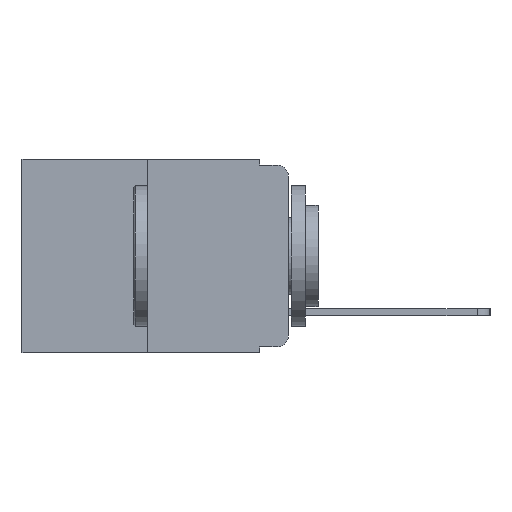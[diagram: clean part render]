
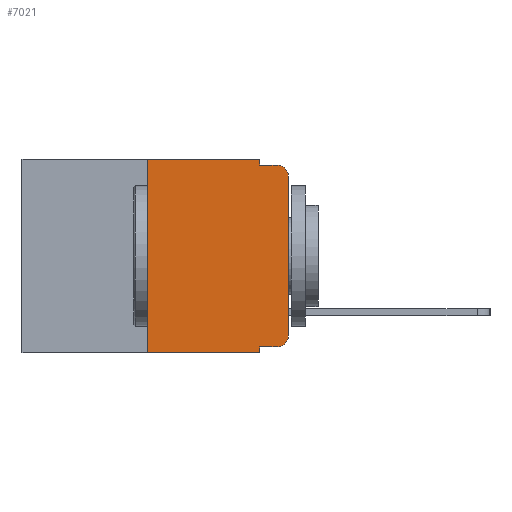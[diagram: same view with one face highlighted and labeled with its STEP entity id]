
A CAD part, left-side view. The second image highlights one B-rep face of the part: STEP entity #7021.
In plain terms, the highlighted planar face has unit normal (-1, 0, 0).
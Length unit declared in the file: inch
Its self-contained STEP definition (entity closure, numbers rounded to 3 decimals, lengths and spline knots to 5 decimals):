
#21 = CARTESIAN_POINT ( 'NONE',  ( 0., 0.473, 0. ) ) ;
#171 = LINE ( 'NONE', #21, #10136 ) ;
#456 = LINE ( 'NONE', #12877, #19580 ) ;
#613 = EDGE_CURVE ( 'NONE', #20553, #6563, #11273, .T. ) ;
#792 = VECTOR ( 'NONE', #21512, 39.37008 ) ;
#1247 = DIRECTION ( 'NONE',  ( 0., 0., -1. ) ) ;
#1403 = VERTEX_POINT ( 'NONE', #15650 ) ;
#1652 = VERTEX_POINT ( 'NONE', #16987 ) ;
#2051 = CARTESIAN_POINT ( 'NONE',  ( 0., 0.02, -0.01 ) ) ;
#2196 = VERTEX_POINT ( 'NONE', #22762 ) ;
#2244 = LINE ( 'NONE', #10944, #20990 ) ;
#2334 = ORIENTED_EDGE ( 'NONE', *, *, #5971, .T. ) ;
#3184 = CARTESIAN_POINT ( 'NONE',  ( 0., 0.473, 0. ) ) ;
#3349 = EDGE_CURVE ( 'NONE', #6563, #7145, #6574, .T. ) ;
#3550 = ORIENTED_EDGE ( 'NONE', *, *, #4656, .T. ) ;
#3631 = ORIENTED_EDGE ( 'NONE', *, *, #3349, .F. ) ;
#4011 = CARTESIAN_POINT ( 'NONE',  ( 0., 0.051, 0. ) ) ;
#4197 = ORIENTED_EDGE ( 'NONE', *, *, #613, .F. ) ;
#4545 = ORIENTED_EDGE ( 'NONE', *, *, #21954, .F. ) ;
#4577 = VERTEX_POINT ( 'NONE', #6796 ) ;
#4656 = EDGE_CURVE ( 'NONE', #1403, #7145, #19176, .T. ) ;
#4668 = CIRCLE ( 'NONE', #15121, 0.02 ) ;
#4827 = ORIENTED_EDGE ( 'NONE', *, *, #23019, .F. ) ;
#5503 = VECTOR ( 'NONE', #15270, 39.37008 ) ;
#5971 = EDGE_CURVE ( 'NONE', #4577, #1403, #456, .T. ) ;
#6563 = VERTEX_POINT ( 'NONE', #11843 ) ;
#6574 = LINE ( 'NONE', #14524, #15285 ) ;
#6796 = CARTESIAN_POINT ( 'NONE',  ( 0., 0., -0.313 ) ) ;
#7021 = ADVANCED_FACE ( 'NONE', ( #13172 ), #10960, .F. ) ;
#7145 = VERTEX_POINT ( 'NONE', #2051 ) ;
#7792 = CARTESIAN_POINT ( 'NONE',  ( 0., 0.25, 0. ) ) ;
#7992 = ORIENTED_EDGE ( 'NONE', *, *, #18848, .T. ) ;
#8192 = CARTESIAN_POINT ( 'NONE',  ( 0., 0.051, -0.333 ) ) ;
#9340 = VERTEX_POINT ( 'NONE', #14673 ) ;
#9566 = CARTESIAN_POINT ( 'NONE',  ( 0., 0.02, -0.03 ) ) ;
#9825 = ORIENTED_EDGE ( 'NONE', *, *, #21900, .F. ) ;
#9887 = LINE ( 'NONE', #8192, #17592 ) ;
#10136 = VECTOR ( 'NONE', #13565, 39.37008 ) ;
#10146 = DIRECTION ( 'NONE',  ( 0., -1., 0. ) ) ;
#10160 = CARTESIAN_POINT ( 'NONE',  ( 0., 0.25, -0.343 ) ) ;
#10360 = DIRECTION ( 'NONE',  ( -1., 0., 0. ) ) ;
#10528 = ORIENTED_EDGE ( 'NONE', *, *, #20785, .T. ) ;
#10809 = VERTEX_POINT ( 'NONE', #12476 ) ;
#10944 = CARTESIAN_POINT ( 'NONE',  ( 0., 0.473, -0.343 ) ) ;
#10960 = PLANE ( 'NONE',  #18819 ) ;
#11174 = DIRECTION ( 'NONE',  ( 0., 0., 1. ) ) ;
#11273 = LINE ( 'NONE', #21348, #792 ) ;
#11479 = DIRECTION ( 'NONE',  ( 0., 0., -1. ) ) ;
#11843 = CARTESIAN_POINT ( 'NONE',  ( 0., 0.051, -0.01 ) ) ;
#12476 = CARTESIAN_POINT ( 'NONE',  ( 0., 0.25, 0. ) ) ;
#12839 = DIRECTION ( 'NONE',  ( 1., 0., 0. ) ) ;
#12877 = CARTESIAN_POINT ( 'NONE',  ( 0., 0., 0. ) ) ;
#12903 = AXIS2_PLACEMENT_3D ( 'NONE', #9566, #21652, #11479 ) ;
#13075 = ORIENTED_EDGE ( 'NONE', *, *, #19672, .T. ) ;
#13172 = FACE_OUTER_BOUND ( 'NONE', #21481, .T. ) ;
#13331 = DIRECTION ( 'NONE',  ( 0., 0., 1. ) ) ;
#13565 = DIRECTION ( 'NONE',  ( 0., -1., 0. ) ) ;
#13749 = VECTOR ( 'NONE', #13331, 39.37008 ) ;
#14524 = CARTESIAN_POINT ( 'NONE',  ( 0., 0.051, -0.01 ) ) ;
#14673 = CARTESIAN_POINT ( 'NONE',  ( 0., 0.051, -0.333 ) ) ;
#15121 = AXIS2_PLACEMENT_3D ( 'NONE', #20646, #10360, #22342 ) ;
#15270 = DIRECTION ( 'NONE',  ( 0., 0., -1. ) ) ;
#15285 = VECTOR ( 'NONE', #16335, 39.37008 ) ;
#15650 = CARTESIAN_POINT ( 'NONE',  ( 0., 0., -0.03 ) ) ;
#15949 = VERTEX_POINT ( 'NONE', #10160 ) ;
#16335 = DIRECTION ( 'NONE',  ( 0., -1., 0. ) ) ;
#16987 = CARTESIAN_POINT ( 'NONE',  ( 0., 0.051, -0.343 ) ) ;
#17592 = VECTOR ( 'NONE', #10146, 39.37008 ) ;
#17930 = DIRECTION ( 'NONE',  ( 0., -1., 0. ) ) ;
#18311 = LINE ( 'NONE', #7792, #13749 ) ;
#18528 = CARTESIAN_POINT ( 'NONE',  ( 0., 0.051, 0. ) ) ;
#18819 = AXIS2_PLACEMENT_3D ( 'NONE', #3184, #12839, #1247 ) ;
#18848 = EDGE_CURVE ( 'NONE', #15949, #1652, #2244, .T. ) ;
#19176 = CIRCLE ( 'NONE', #12903, 0.02 ) ;
#19580 = VECTOR ( 'NONE', #11174, 39.37008 ) ;
#19672 = EDGE_CURVE ( 'NONE', #2196, #4577, #4668, .T. ) ;
#20395 = LINE ( 'NONE', #4011, #5503 ) ;
#20553 = VERTEX_POINT ( 'NONE', #18528 ) ;
#20646 = CARTESIAN_POINT ( 'NONE',  ( 0., 0.02, -0.313 ) ) ;
#20785 = EDGE_CURVE ( 'NONE', #9340, #2196, #9887, .T. ) ;
#20990 = VECTOR ( 'NONE', #17930, 39.37008 ) ;
#21348 = CARTESIAN_POINT ( 'NONE',  ( 0., 0.051, 0. ) ) ;
#21481 = EDGE_LOOP ( 'NONE', ( #2334, #3550, #3631, #4197, #4545, #4827, #7992, #9825, #10528, #13075 ) ) ;
#21512 = DIRECTION ( 'NONE',  ( 0., 0., -1. ) ) ;
#21652 = DIRECTION ( 'NONE',  ( -1., 0., 0. ) ) ;
#21900 = EDGE_CURVE ( 'NONE', #9340, #1652, #20395, .T. ) ;
#21954 = EDGE_CURVE ( 'NONE', #10809, #20553, #171, .T. ) ;
#22342 = DIRECTION ( 'NONE',  ( 0., 0., -1. ) ) ;
#22762 = CARTESIAN_POINT ( 'NONE',  ( 0., 0.02, -0.333 ) ) ;
#23019 = EDGE_CURVE ( 'NONE', #15949, #10809, #18311, .T. ) ;
